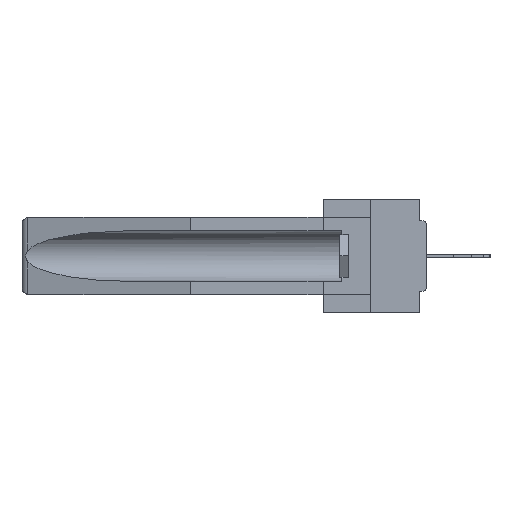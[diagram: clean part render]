
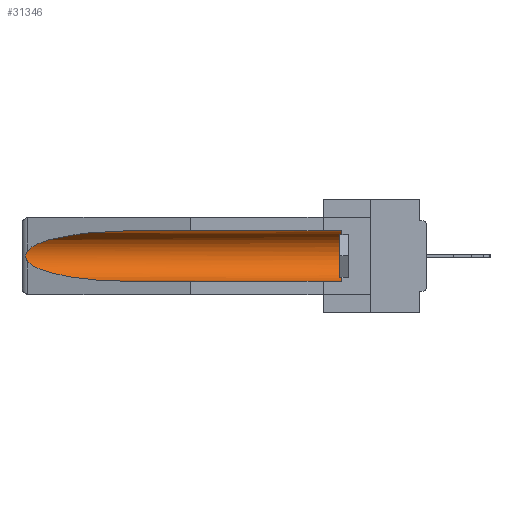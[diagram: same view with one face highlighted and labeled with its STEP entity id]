
A CAD part, left-side view. The second image highlights one B-rep face of the part: STEP entity #31346.
In plain terms, the highlighted cylindrical face has radius 2.857 mm (diameter 5.715 mm), a partial arc.
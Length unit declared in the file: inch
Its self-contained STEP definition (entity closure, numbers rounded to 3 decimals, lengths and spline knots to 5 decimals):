
#1307 = CARTESIAN_POINT ( 'NONE',  ( 0.2675, 1.53308, -0.16763 ) ) ;
#1346 = VERTEX_POINT ( 'NONE', #11168 ) ;
#1387 = ORIENTED_EDGE ( 'NONE', *, *, #28438, .T. ) ;
#1575 = DIRECTION ( 'NONE',  ( 0., -1., 0. ) ) ;
#2374 = EDGE_CURVE ( 'NONE', #30198, #5577, #32964, .T. ) ;
#3080 = CARTESIAN_POINT ( 'NONE',  ( 0.26537, 1.52718, -0.14972 ) ) ;
#5073 = CARTESIAN_POINT ( 'NONE',  ( 0.155, -0.30754, -0.284 ) ) ;
#5577 = VERTEX_POINT ( 'NONE', #38711 ) ;
#5703 = CARTESIAN_POINT ( 'NONE',  ( 0.25451, 1.48313, -0.09465 ) ) ;
#6097 = CARTESIAN_POINT ( 'NONE',  ( 0.26537, 1.52718, -0.14972 ) ) ;
#7022 = CARTESIAN_POINT ( 'NONE',  ( 0.155, -0.30754, -0.059 ) ) ;
#8898 = CARTESIAN_POINT ( 'NONE',  ( 0.155, 1.07973, -0.059 ) ) ;
#10510 = CARTESIAN_POINT ( 'NONE',  ( 0.2673, 1.5327, -0.16383 ) ) ;
#10977 = DIRECTION ( 'NONE',  ( 0., 0., 1. ) ) ;
#11168 = CARTESIAN_POINT ( 'NONE',  ( 0.155, 1.07973, -0.059 ) ) ;
#11999 = CARTESIAN_POINT ( 'NONE',  ( 0.26537, 1.52718, -0.19328 ) ) ;
#12735 = ORIENTED_EDGE ( 'NONE', *, *, #35177, .T. ) ;
#12785 = EDGE_LOOP ( 'NONE', ( #1387, #36505, #23800, #16167, #12735, #35516 ) ) ;
#13494 = CYLINDRICAL_SURFACE ( 'NONE', #32224, 0.1125 ) ;
#13854 = CARTESIAN_POINT ( 'NONE',  ( 0.26537, 1.52718, -0.14972 ) ) ;
#13881 = CIRCLE ( 'NONE', #18992, 0.1125 ) ;
#14103 = CARTESIAN_POINT ( 'NONE',  ( 0.21114, 1.30732, -0.284 ) ) ;
#15721 = VECTOR ( 'NONE', #23636, 39.37008 ) ;
#16167 = ORIENTED_EDGE ( 'NONE', *, *, #2374, .F. ) ;
#16292 = DIRECTION ( 'NONE',  ( 0., 1., 0. ) ) ;
#17851 = EDGE_CURVE ( 'NONE', #18928, #1346, #25374, .T. ) ;
#18928 = VERTEX_POINT ( 'NONE', #22866 ) ;
#18992 = AXIS2_PLACEMENT_3D ( 'NONE', #29122, #1575, #10977 ) ;
#19692 = EDGE_CURVE ( 'NONE', #31879, #5577, #29573, .T. ) ;
#20070 = FACE_OUTER_BOUND ( 'NONE', #12785, .T. ) ;
#20497 = CARTESIAN_POINT ( 'NONE',  ( 0.26537, 1.52718, -0.19328 ) ) ;
#21611 = EDGE_CURVE ( 'NONE', #37466, #31879, #37250, .T. ) ;
#22467 = CARTESIAN_POINT ( 'NONE',  ( 0.26654, 1.53092, -0.15636 ) ) ;
#22659 = CARTESIAN_POINT ( 'NONE',  ( 0.2673, 1.53269, -0.17917 ) ) ;
#22862 = CARTESIAN_POINT ( 'NONE',  ( 0.26597, 1.52961, -0.15275 ) ) ;
#22866 = CARTESIAN_POINT ( 'NONE',  ( 0.155, 0.126, -0.059 ) ) ;
#23058 = CARTESIAN_POINT ( 'NONE',  ( 0.26537, 1.52718, -0.19328 ) ) ;
#23636 = DIRECTION ( 'NONE',  ( 0., 1., 0. ) ) ;
#23800 = ORIENTED_EDGE ( 'NONE', *, *, #19692, .T. ) ;
#25374 = LINE ( 'NONE', #7022, #33159 ) ;
#25700 = DIRECTION ( 'NONE',  ( 0., 0., 1. ) ) ;
#28438 = EDGE_CURVE ( 'NONE', #1346, #37466, #32570, .T. ) ;
#29078 = CARTESIAN_POINT ( 'NONE',  ( 0.155, -0.30754, -0.1715 ) ) ;
#29122 = CARTESIAN_POINT ( 'NONE',  ( 0.155, 0.126, -0.1715 ) ) ;
#29573 =( BOUNDED_CURVE ( )  B_SPLINE_CURVE ( 3, ( #20497, #31870, #14103, #38035 ),
 .UNSPECIFIED., .F., .F. ) 
 B_SPLINE_CURVE_WITH_KNOTS ( ( 4, 4 ),
 ( 0.1948, 1.5708 ),
 .UNSPECIFIED. ) 
 CURVE ( )  GEOMETRIC_REPRESENTATION_ITEM ( )  RATIONAL_B_SPLINE_CURVE ( ( 1., 0.848, 0.848, 1. ) ) 
 REPRESENTATION_ITEM ( '' )  );
#30033 = CARTESIAN_POINT ( 'NONE',  ( 0.21114, 1.30732, -0.059 ) ) ;
#30198 = VERTEX_POINT ( 'NONE', #38927 ) ;
#31346 = ADVANCED_FACE ( 'NONE', ( #20070 ), #13494, .F. ) ;
#31720 = DIRECTION ( 'NONE',  ( 0., 1., 0. ) ) ;
#31870 = CARTESIAN_POINT ( 'NONE',  ( 0.25451, 1.48313, -0.24835 ) ) ;
#31879 = VERTEX_POINT ( 'NONE', #11999 ) ;
#32011 = CARTESIAN_POINT ( 'NONE',  ( 0.26655, 1.53094, -0.18657 ) ) ;
#32224 = AXIS2_PLACEMENT_3D ( 'NONE', #29078, #16292, #25700 ) ;
#32399 = CARTESIAN_POINT ( 'NONE',  ( 0.26597, 1.5296, -0.19026 ) ) ;
#32570 =( BOUNDED_CURVE ( )  B_SPLINE_CURVE ( 3, ( #8898, #30033, #5703, #6097 ),
 .UNSPECIFIED., .F., .F. ) 
 B_SPLINE_CURVE_WITH_KNOTS ( ( 4, 4 ),
 ( 4.71239, 6.08839 ),
 .UNSPECIFIED. ) 
 CURVE ( )  GEOMETRIC_REPRESENTATION_ITEM ( )  RATIONAL_B_SPLINE_CURVE ( ( 1., 0.848, 0.848, 1. ) ) 
 REPRESENTATION_ITEM ( '' )  );
#32964 = LINE ( 'NONE', #5073, #15721 ) ;
#33159 = VECTOR ( 'NONE', #31720, 39.37008 ) ;
#34985 = CARTESIAN_POINT ( 'NONE',  ( 0.2675, 1.53308, -0.17534 ) ) ;
#35177 = EDGE_CURVE ( 'NONE', #30198, #18928, #13881, .T. ) ;
#35516 = ORIENTED_EDGE ( 'NONE', *, *, #17851, .T. ) ;
#36505 = ORIENTED_EDGE ( 'NONE', *, *, #21611, .T. ) ;
#37250 = B_SPLINE_CURVE_WITH_KNOTS ( 'NONE', 3,
 ( #13854, #22862, #22467, #10510, #1307, #34985, #22659, #32011, #32399, #23058 ),
 .UNSPECIFIED., .F., .F.,
 ( 4, 2, 2, 2, 4 ),
 ( 0., 0.00029, 0.00058, 0.00087, 0.00117 ),
 .UNSPECIFIED. ) ;
#37466 = VERTEX_POINT ( 'NONE', #3080 ) ;
#38035 = CARTESIAN_POINT ( 'NONE',  ( 0.155, 1.07973, -0.284 ) ) ;
#38711 = CARTESIAN_POINT ( 'NONE',  ( 0.155, 1.07973, -0.284 ) ) ;
#38927 = CARTESIAN_POINT ( 'NONE',  ( 0.155, 0.126, -0.284 ) ) ;
